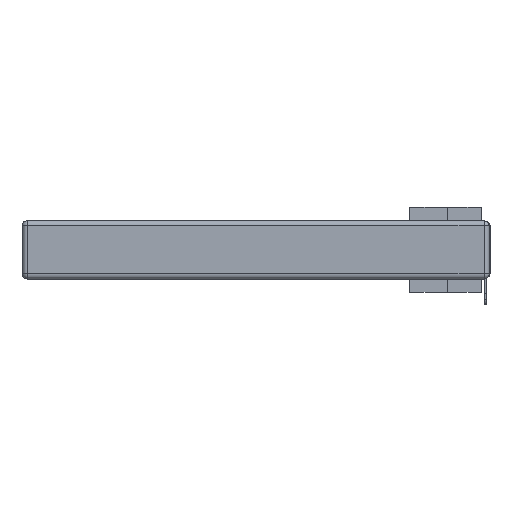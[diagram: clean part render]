
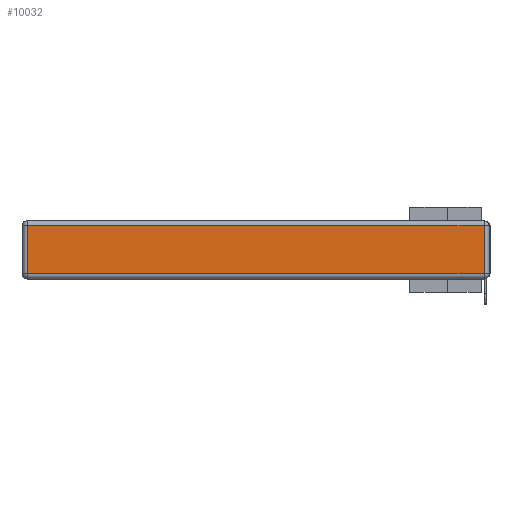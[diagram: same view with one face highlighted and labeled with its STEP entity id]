
A CAD part, left-side view. The second image highlights one B-rep face of the part: STEP entity #10032.
In plain terms, the highlighted planar face has unit normal (-1, 0, 0).
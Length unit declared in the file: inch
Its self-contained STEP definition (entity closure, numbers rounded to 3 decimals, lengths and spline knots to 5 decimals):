
#1147 = ORIENTED_EDGE ( 'NONE', *, *, #21046, .T. ) ;
#1360 = DIRECTION ( 'NONE',  ( 0., 0., 1. ) ) ;
#2955 = DIRECTION ( 'NONE',  ( 0., 0., 1. ) ) ;
#5020 = DIRECTION ( 'NONE',  ( 0., -1., 0. ) ) ;
#5401 = CARTESIAN_POINT ( 'NONE',  ( 0., 2.72, -0.03 ) ) ;
#5606 = PLANE ( 'NONE',  #8058 ) ;
#5923 = VECTOR ( 'NONE', #29013, 39.37008 ) ;
#8058 = AXIS2_PLACEMENT_3D ( 'NONE', #38015, #28252, #2955 ) ;
#9296 = VERTEX_POINT ( 'NONE', #27335 ) ;
#10032 = ADVANCED_FACE ( 'NONE', ( #32677 ), #5606, .T. ) ;
#10621 = DIRECTION ( 'NONE',  ( 0., 0., -1. ) ) ;
#11745 = ORIENTED_EDGE ( 'NONE', *, *, #18843, .T. ) ;
#13520 = LINE ( 'NONE', #20130, #25474 ) ;
#14577 = CARTESIAN_POINT ( 'NONE',  ( 0., 0., -0.313 ) ) ;
#16355 = CARTESIAN_POINT ( 'NONE',  ( 0., 2.75, -0.03 ) ) ;
#18843 = EDGE_CURVE ( 'NONE', #24527, #19153, #35785, .T. ) ;
#19153 = VERTEX_POINT ( 'NONE', #5401 ) ;
#19249 = CARTESIAN_POINT ( 'NONE',  ( 0., 0.03, -0.313 ) ) ;
#20130 = CARTESIAN_POINT ( 'NONE',  ( 0., 2.72, -0.343 ) ) ;
#21046 = EDGE_CURVE ( 'NONE', #19153, #9296, #13520, .T. ) ;
#21315 = VERTEX_POINT ( 'NONE', #19249 ) ;
#21721 = LINE ( 'NONE', #29656, #22245 ) ;
#22245 = VECTOR ( 'NONE', #1360, 39.37008 ) ;
#23069 = EDGE_LOOP ( 'NONE', ( #37987, #29411, #11745, #1147 ) ) ;
#24527 = VERTEX_POINT ( 'NONE', #27270 ) ;
#25474 = VECTOR ( 'NONE', #10621, 39.37008 ) ;
#26651 = VECTOR ( 'NONE', #5020, 39.37008 ) ;
#27270 = CARTESIAN_POINT ( 'NONE',  ( 0., 0.03, -0.03 ) ) ;
#27311 = EDGE_CURVE ( 'NONE', #21315, #24527, #21721, .T. ) ;
#27335 = CARTESIAN_POINT ( 'NONE',  ( 0., 2.72, -0.313 ) ) ;
#28252 = DIRECTION ( 'NONE',  ( -1., 0., 0. ) ) ;
#29013 = DIRECTION ( 'NONE',  ( 0., 1., 0. ) ) ;
#29411 = ORIENTED_EDGE ( 'NONE', *, *, #27311, .T. ) ;
#29656 = CARTESIAN_POINT ( 'NONE',  ( 0., 0.03, -0.343 ) ) ;
#30638 = LINE ( 'NONE', #14577, #26651 ) ;
#32677 = FACE_OUTER_BOUND ( 'NONE', #23069, .T. ) ;
#35785 = LINE ( 'NONE', #16355, #5923 ) ;
#37141 = EDGE_CURVE ( 'NONE', #9296, #21315, #30638, .T. ) ;
#37987 = ORIENTED_EDGE ( 'NONE', *, *, #37141, .T. ) ;
#38015 = CARTESIAN_POINT ( 'NONE',  ( 0., 0., -0.343 ) ) ;
